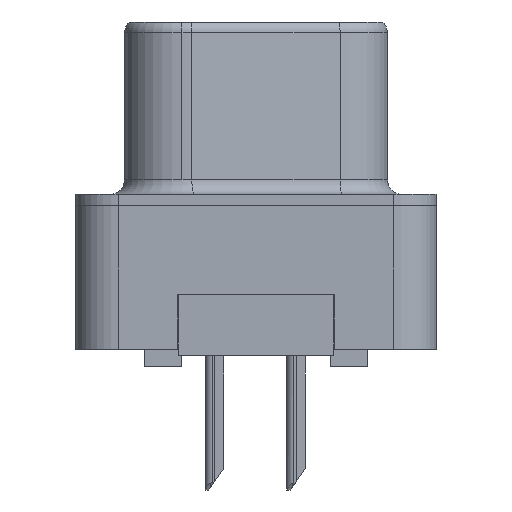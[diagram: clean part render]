
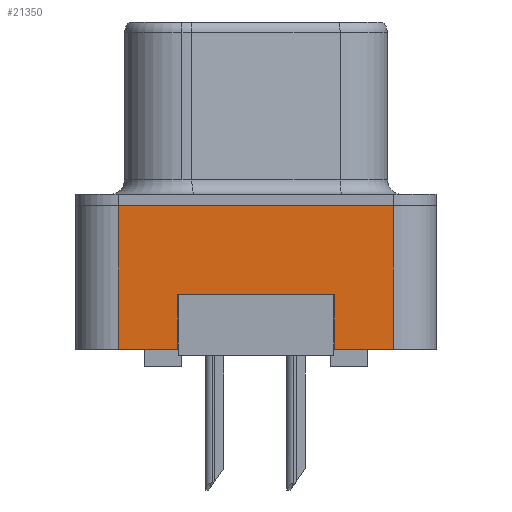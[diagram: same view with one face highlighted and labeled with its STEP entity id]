
A CAD part, left-side view. The second image highlights one B-rep face of the part: STEP entity #21350.
In plain terms, the highlighted planar face has unit normal (-1, 0, 0).
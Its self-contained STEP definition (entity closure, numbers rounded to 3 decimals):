
#104 = DIRECTION ( 'NONE',  ( 0., 0., 1. ) ) ;
#159 = VECTOR ( 'NONE', #18094, 1000. ) ;
#1214 = DIRECTION ( 'NONE',  ( 0., -1., 0. ) ) ;
#1314 = LINE ( 'NONE', #19452, #27911 ) ;
#1442 = ORIENTED_EDGE ( 'NONE', *, *, #14714, .F. ) ;
#1571 = CARTESIAN_POINT ( 'NONE',  ( -2.91, -4.775, -5. ) ) ;
#1586 = VECTOR ( 'NONE', #14921, 1000. ) ;
#2059 = LINE ( 'NONE', #11530, #159 ) ;
#2764 = LINE ( 'NONE', #13747, #13247 ) ;
#2992 = EDGE_CURVE ( 'NONE', #24421, #7084, #1314, .T. ) ;
#3096 = EDGE_CURVE ( 'NONE', #21656, #14707, #2059, .T. ) ;
#3225 = VERTEX_POINT ( 'NONE', #28118 ) ;
#3396 = CARTESIAN_POINT ( 'NONE',  ( -2.91, 4.775, -5. ) ) ;
#3842 = DIRECTION ( 'NONE',  ( 0., 1., 0. ) ) ;
#3867 = VERTEX_POINT ( 'NONE', #13513 ) ;
#3953 = ORIENTED_EDGE ( 'NONE', *, *, #2992, .T. ) ;
#5180 = VECTOR ( 'NONE', #1214, 1000. ) ;
#6711 = DIRECTION ( 'NONE',  ( 0., -1., 0. ) ) ;
#7084 = VERTEX_POINT ( 'NONE', #25900 ) ;
#7780 = CARTESIAN_POINT ( 'NONE',  ( -2.91, -2.75, -3.1 ) ) ;
#8301 = CARTESIAN_POINT ( 'NONE',  ( -2.91, -4.775, -5. ) ) ;
#8666 = DIRECTION ( 'NONE',  ( 0., 0., 1. ) ) ;
#8961 = LINE ( 'NONE', #27241, #12571 ) ;
#11011 = DIRECTION ( 'NONE',  ( 0., 0., 1. ) ) ;
#11186 = EDGE_CURVE ( 'NONE', #18050, #3867, #15732, .T. ) ;
#11530 = CARTESIAN_POINT ( 'NONE',  ( -2.91, -2.75, -3.1 ) ) ;
#12571 = VECTOR ( 'NONE', #6711, 1000. ) ;
#13247 = VECTOR ( 'NONE', #104, 1000. ) ;
#13513 = CARTESIAN_POINT ( 'NONE',  ( -2.91, 2.75, -5. ) ) ;
#13747 = CARTESIAN_POINT ( 'NONE',  ( -2.91, 4.775, -5. ) ) ;
#14419 = CARTESIAN_POINT ( 'NONE',  ( -2.91, 2.75, -3.1 ) ) ;
#14707 = VERTEX_POINT ( 'NONE', #26401 ) ;
#14714 = EDGE_CURVE ( 'NONE', #3225, #7084, #19499, .T. ) ;
#14921 = DIRECTION ( 'NONE',  ( 0., -1., 0. ) ) ;
#15353 = PLANE ( 'NONE',  #19016 ) ;
#15435 = CARTESIAN_POINT ( 'NONE',  ( -2.91, 2.75, -3.1 ) ) ;
#15732 = LINE ( 'NONE', #15435, #26056 ) ;
#16854 = EDGE_CURVE ( 'NONE', #21656, #18050, #29182, .T. ) ;
#17968 = CARTESIAN_POINT ( 'NONE',  ( -2.91, -4.775, -5. ) ) ;
#18050 = VERTEX_POINT ( 'NONE', #14419 ) ;
#18094 = DIRECTION ( 'NONE',  ( 0., 0., -1. ) ) ;
#18378 = ORIENTED_EDGE ( 'NONE', *, *, #28442, .T. ) ;
#19016 = AXIS2_PLACEMENT_3D ( 'NONE', #8301, #29120, #11011 ) ;
#19452 = CARTESIAN_POINT ( 'NONE',  ( -2.91, -4.775, -5. ) ) ;
#19499 = LINE ( 'NONE', #26106, #5180 ) ;
#20024 = EDGE_LOOP ( 'NONE', ( #24135, #25354, #3953, #1442, #23031, #18378, #28068, #22884 ) ) ;
#21063 = EDGE_CURVE ( 'NONE', #28109, #3225, #2764, .T. ) ;
#21350 = ADVANCED_FACE ( 'NONE', ( #22523 ), #15353, .T. ) ;
#21656 = VERTEX_POINT ( 'NONE', #7780 ) ;
#21689 = CARTESIAN_POINT ( 'NONE',  ( -2.91, 2.75, -3.1 ) ) ;
#22523 = FACE_OUTER_BOUND ( 'NONE', #20024, .T. ) ;
#22884 = ORIENTED_EDGE ( 'NONE', *, *, #16854, .F. ) ;
#23031 = ORIENTED_EDGE ( 'NONE', *, *, #21063, .F. ) ;
#24135 = ORIENTED_EDGE ( 'NONE', *, *, #3096, .T. ) ;
#24421 = VERTEX_POINT ( 'NONE', #17968 ) ;
#24423 = VECTOR ( 'NONE', #3842, 1000. ) ;
#25354 = ORIENTED_EDGE ( 'NONE', *, *, #28690, .T. ) ;
#25900 = CARTESIAN_POINT ( 'NONE',  ( -2.91, -4.775, 0. ) ) ;
#26056 = VECTOR ( 'NONE', #28762, 1000. ) ;
#26106 = CARTESIAN_POINT ( 'NONE',  ( -2.91, -4.775, 0. ) ) ;
#26401 = CARTESIAN_POINT ( 'NONE',  ( -2.91, -2.75, -5. ) ) ;
#27241 = CARTESIAN_POINT ( 'NONE',  ( -2.91, -4.775, -5. ) ) ;
#27911 = VECTOR ( 'NONE', #8666, 1000. ) ;
#28068 = ORIENTED_EDGE ( 'NONE', *, *, #11186, .F. ) ;
#28109 = VERTEX_POINT ( 'NONE', #3396 ) ;
#28118 = CARTESIAN_POINT ( 'NONE',  ( -2.91, 4.775, 0. ) ) ;
#28442 = EDGE_CURVE ( 'NONE', #28109, #3867, #8961, .T. ) ;
#28690 = EDGE_CURVE ( 'NONE', #14707, #24421, #28852, .T. ) ;
#28762 = DIRECTION ( 'NONE',  ( 0., 0., -1. ) ) ;
#28852 = LINE ( 'NONE', #1571, #1586 ) ;
#29120 = DIRECTION ( 'NONE',  ( -1., 0., 0. ) ) ;
#29182 = LINE ( 'NONE', #21689, #24423 ) ;
